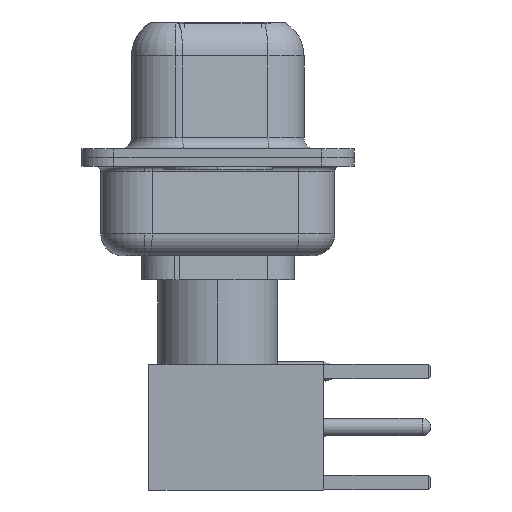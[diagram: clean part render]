
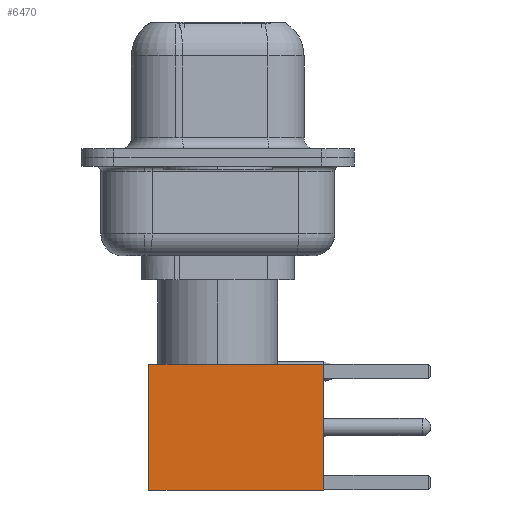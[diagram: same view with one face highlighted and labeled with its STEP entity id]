
A CAD part, left-side view. The second image highlights one B-rep face of the part: STEP entity #6470.
In plain terms, the highlighted face is planar.
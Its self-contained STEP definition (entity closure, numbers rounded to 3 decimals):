
#1110 = FACE_OUTER_BOUND ( 'NONE', #2634, .T. ) ;
#2095 = VECTOR ( 'NONE', #9850, 1000. ) ;
#2307 = VERTEX_POINT ( 'NONE', #7413 ) ;
#2634 = EDGE_LOOP ( 'NONE', ( #14712, #18154, #16661, #13780 ) ) ;
#4388 = EDGE_CURVE ( 'NONE', #19434, #22551, #5685, .T. ) ;
#5105 = AXIS2_PLACEMENT_3D ( 'NONE', #25166, #14757, #9302 ) ;
#5555 = EDGE_CURVE ( 'NONE', #17514, #2307, #21195, .T. ) ;
#5685 = LINE ( 'NONE', #12036, #2095 ) ;
#6470 = ADVANCED_FACE ( 'NONE', ( #1110 ), #14886, .T. ) ;
#6899 = CARTESIAN_POINT ( 'NONE',  ( 0., 2.875, 0. ) ) ;
#7386 = VECTOR ( 'NONE', #12848, 1000. ) ;
#7413 = CARTESIAN_POINT ( 'NONE',  ( -2.875, 2.875, 0. ) ) ;
#8471 = DIRECTION ( 'NONE',  ( -1., 0., 0. ) ) ;
#8730 = LINE ( 'NONE', #6899, #7386 ) ;
#9302 = DIRECTION ( 'NONE',  ( 0., 0., 1. ) ) ;
#9850 = DIRECTION ( 'NONE',  ( 0., 0., -1. ) ) ;
#10307 = VECTOR ( 'NONE', #8471, 1000. ) ;
#12036 = CARTESIAN_POINT ( 'NONE',  ( 2.875, 2.875, 0. ) ) ;
#12048 = EDGE_CURVE ( 'NONE', #19434, #17514, #15127, .T. ) ;
#12848 = DIRECTION ( 'NONE',  ( -1., 0., 0. ) ) ;
#13116 = CARTESIAN_POINT ( 'NONE',  ( -2.875, 2.875, 0. ) ) ;
#13780 = ORIENTED_EDGE ( 'NONE', *, *, #12048, .F. ) ;
#14712 = ORIENTED_EDGE ( 'NONE', *, *, #4388, .T. ) ;
#14757 = DIRECTION ( 'NONE',  ( 0., 1., 0. ) ) ;
#14886 = PLANE ( 'NONE',  #5105 ) ;
#15127 = LINE ( 'NONE', #18199, #10307 ) ;
#16661 = ORIENTED_EDGE ( 'NONE', *, *, #5555, .F. ) ;
#17514 = VERTEX_POINT ( 'NONE', #23552 ) ;
#18154 = ORIENTED_EDGE ( 'NONE', *, *, #20526, .T. ) ;
#18199 = CARTESIAN_POINT ( 'NONE',  ( 0., 2.875, 8. ) ) ;
#19434 = VERTEX_POINT ( 'NONE', #24432 ) ;
#20526 = EDGE_CURVE ( 'NONE', #22551, #2307, #8730, .T. ) ;
#21162 = CARTESIAN_POINT ( 'NONE',  ( 2.875, 2.875, 0. ) ) ;
#21195 = LINE ( 'NONE', #13116, #21647 ) ;
#21647 = VECTOR ( 'NONE', #25235, 1000. ) ;
#22551 = VERTEX_POINT ( 'NONE', #21162 ) ;
#23552 = CARTESIAN_POINT ( 'NONE',  ( -2.875, 2.875, 8. ) ) ;
#24432 = CARTESIAN_POINT ( 'NONE',  ( 2.875, 2.875, 8. ) ) ;
#25166 = CARTESIAN_POINT ( 'NONE',  ( 2.875, 2.875, 0. ) ) ;
#25235 = DIRECTION ( 'NONE',  ( 0., 0., -1. ) ) ;
